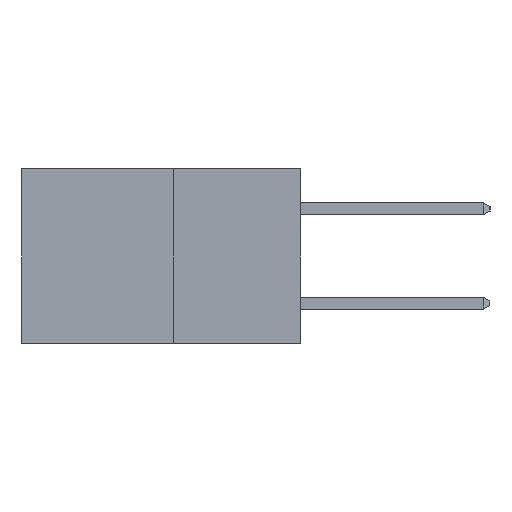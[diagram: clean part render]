
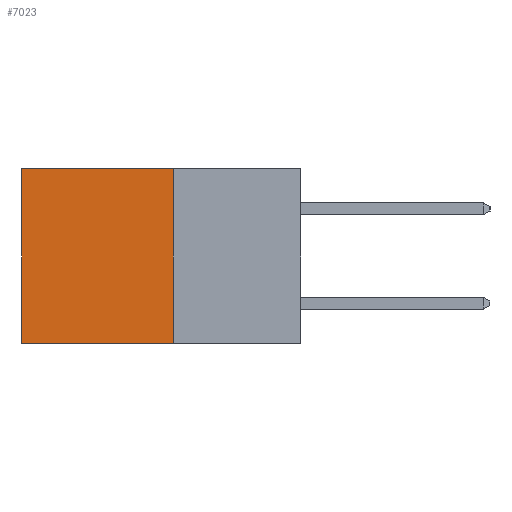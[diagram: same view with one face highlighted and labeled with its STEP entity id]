
A CAD part, left-side view. The second image highlights one B-rep face of the part: STEP entity #7023.
In plain terms, the highlighted planar face has unit normal (-1, 0, 0).
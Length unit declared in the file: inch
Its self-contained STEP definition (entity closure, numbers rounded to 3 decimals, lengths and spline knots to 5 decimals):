
#176 = EDGE_LOOP ( 'NONE', ( #9058, #19085, #22731, #22508 ) ) ;
#3180 = EDGE_CURVE ( 'NONE', #29166, #32103, #19652, .T. ) ;
#3748 = LINE ( 'NONE', #27481, #16439 ) ;
#5602 = VECTOR ( 'NONE', #5751, 39.37008 ) ;
#5751 = DIRECTION ( 'NONE',  ( 0., 1., 0. ) ) ;
#7023 = ADVANCED_FACE ( 'NONE', ( #25408 ), #7048, .F. ) ;
#7048 = PLANE ( 'NONE',  #21610 ) ;
#9051 = EDGE_CURVE ( 'NONE', #15139, #10164, #3748, .T. ) ;
#9058 = ORIENTED_EDGE ( 'NONE', *, *, #3180, .T. ) ;
#9590 = DIRECTION ( 'NONE',  ( 1., 0., 0. ) ) ;
#10164 = VERTEX_POINT ( 'NONE', #16419 ) ;
#14652 = CARTESIAN_POINT ( 'NONE',  ( 0.277, 0.59, -0.37 ) ) ;
#15139 = VERTEX_POINT ( 'NONE', #28329 ) ;
#16419 = CARTESIAN_POINT ( 'NONE',  ( 0.277, 0.27, -0.37 ) ) ;
#16439 = VECTOR ( 'NONE', #24945, 39.37008 ) ;
#16935 = DIRECTION ( 'NONE',  ( 0., 0., -1. ) ) ;
#17879 = EDGE_CURVE ( 'NONE', #10164, #32103, #17958, .T. ) ;
#17958 = LINE ( 'NONE', #20044, #30596 ) ;
#19085 = ORIENTED_EDGE ( 'NONE', *, *, #17879, .F. ) ;
#19108 = LINE ( 'NONE', #20960, #5602 ) ;
#19652 = LINE ( 'NONE', #14652, #25615 ) ;
#20044 = CARTESIAN_POINT ( 'NONE',  ( 0.277, 0.27, -0.37 ) ) ;
#20960 = CARTESIAN_POINT ( 'NONE',  ( 0.277, 0.27, 0. ) ) ;
#21610 = AXIS2_PLACEMENT_3D ( 'NONE', #22275, #9590, #27374 ) ;
#22275 = CARTESIAN_POINT ( 'NONE',  ( 0.277, 0.27, -0.37 ) ) ;
#22508 = ORIENTED_EDGE ( 'NONE', *, *, #27728, .T. ) ;
#22560 = CARTESIAN_POINT ( 'NONE',  ( 0.277, 0.59, -0.37 ) ) ;
#22731 = ORIENTED_EDGE ( 'NONE', *, *, #9051, .F. ) ;
#24945 = DIRECTION ( 'NONE',  ( 0., 0., -1. ) ) ;
#25408 = FACE_OUTER_BOUND ( 'NONE', #176, .T. ) ;
#25615 = VECTOR ( 'NONE', #16935, 39.37008 ) ;
#26614 = CARTESIAN_POINT ( 'NONE',  ( 0.277, 0.59, 0. ) ) ;
#27374 = DIRECTION ( 'NONE',  ( 0., 0., -1. ) ) ;
#27481 = CARTESIAN_POINT ( 'NONE',  ( 0.277, 0.27, -0.37 ) ) ;
#27728 = EDGE_CURVE ( 'NONE', #15139, #29166, #19108, .T. ) ;
#28329 = CARTESIAN_POINT ( 'NONE',  ( 0.277, 0.27, 0. ) ) ;
#29166 = VERTEX_POINT ( 'NONE', #26614 ) ;
#30596 = VECTOR ( 'NONE', #32576, 39.37008 ) ;
#32103 = VERTEX_POINT ( 'NONE', #22560 ) ;
#32576 = DIRECTION ( 'NONE',  ( 0., 1., 0. ) ) ;
